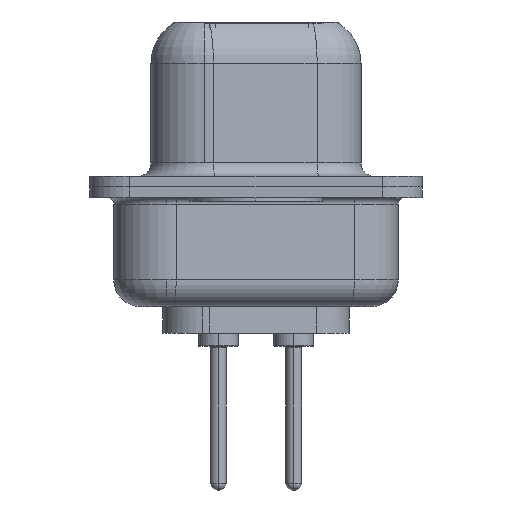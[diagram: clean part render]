
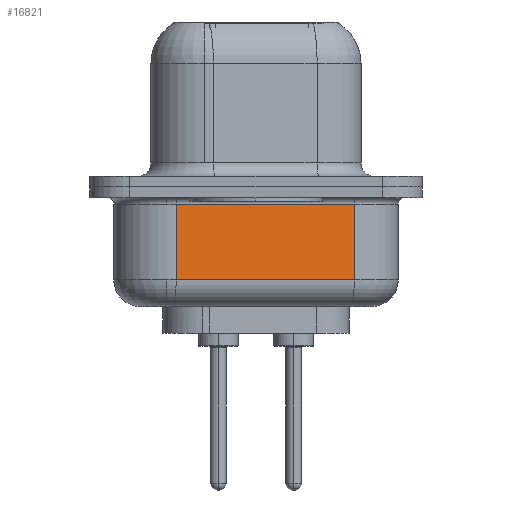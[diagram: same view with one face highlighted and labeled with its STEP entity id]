
A CAD part, left-side view. The second image highlights one B-rep face of the part: STEP entity #16821.
In plain terms, the highlighted planar face has unit normal (-0.985, -0.174, 0).
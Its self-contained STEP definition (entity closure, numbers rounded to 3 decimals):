
#274 = LINE ( 'NONE', #15445, #15747 ) ;
#370 = CARTESIAN_POINT ( 'NONE',  ( 2.855, 3.003, -3.5 ) ) ;
#1943 = ORIENTED_EDGE ( 'NONE', *, *, #9723, .F. ) ;
#2059 = CARTESIAN_POINT ( 'NONE',  ( 4.037, -3.697, -3.5 ) ) ;
#2073 = VERTEX_POINT ( 'NONE', #2059 ) ;
#3429 = ORIENTED_EDGE ( 'NONE', *, *, #14297, .T. ) ;
#4602 = LINE ( 'NONE', #10875, #11607 ) ;
#4819 = VECTOR ( 'NONE', #6530, 1000. ) ;
#5764 = AXIS2_PLACEMENT_3D ( 'NONE', #16584, #8889, #7386 ) ;
#6530 = DIRECTION ( 'NONE',  ( 0.174, -0.985, 0. ) ) ;
#7004 = ORIENTED_EDGE ( 'NONE', *, *, #13234, .T. ) ;
#7216 = VERTEX_POINT ( 'NONE', #14593 ) ;
#7250 = CARTESIAN_POINT ( 'NONE',  ( 4.037, -3.697, -0.65 ) ) ;
#7386 = DIRECTION ( 'NONE',  ( -0.174, 0.985, 0. ) ) ;
#8064 = LINE ( 'NONE', #370, #4819 ) ;
#8805 = ORIENTED_EDGE ( 'NONE', *, *, #19858, .T. ) ;
#8889 = DIRECTION ( 'NONE',  ( 0.985, 0.174, 0. ) ) ;
#9471 = DIRECTION ( 'NONE',  ( 0., 0., 1. ) ) ;
#9723 = EDGE_CURVE ( 'NONE', #7216, #14545, #274, .T. ) ;
#10406 = PLANE ( 'NONE',  #5764 ) ;
#10875 = CARTESIAN_POINT ( 'NONE',  ( 2.855, 3.003, -0.65 ) ) ;
#11607 = VECTOR ( 'NONE', #13832, 1000. ) ;
#11992 = VECTOR ( 'NONE', #13217, 1000. ) ;
#12803 = LINE ( 'NONE', #16256, #11992 ) ;
#13217 = DIRECTION ( 'NONE',  ( 0., 0., 1. ) ) ;
#13234 = EDGE_CURVE ( 'NONE', #7216, #2073, #8064, .T. ) ;
#13832 = DIRECTION ( 'NONE',  ( -0.174, 0.985, 0. ) ) ;
#14297 = EDGE_CURVE ( 'NONE', #2073, #14515, #12803, .T. ) ;
#14515 = VERTEX_POINT ( 'NONE', #7250 ) ;
#14545 = VERTEX_POINT ( 'NONE', #15424 ) ;
#14593 = CARTESIAN_POINT ( 'NONE',  ( 2.855, 3.003, -3.5 ) ) ;
#15424 = CARTESIAN_POINT ( 'NONE',  ( 2.855, 3.003, -0.65 ) ) ;
#15445 = CARTESIAN_POINT ( 'NONE',  ( 2.855, 3.003, -4.5 ) ) ;
#15747 = VECTOR ( 'NONE', #9471, 1000. ) ;
#16256 = CARTESIAN_POINT ( 'NONE',  ( 4.037, -3.697, -4.5 ) ) ;
#16584 = CARTESIAN_POINT ( 'NONE',  ( 2.855, 3.003, -4.5 ) ) ;
#16821 = ADVANCED_FACE ( 'NONE', ( #19605 ), #10406, .F. ) ;
#17811 = EDGE_LOOP ( 'NONE', ( #1943, #7004, #3429, #8805 ) ) ;
#19605 = FACE_OUTER_BOUND ( 'NONE', #17811, .T. ) ;
#19858 = EDGE_CURVE ( 'NONE', #14515, #14545, #4602, .T. ) ;
